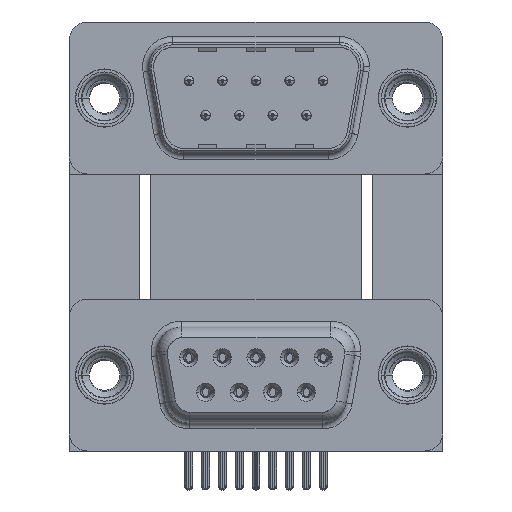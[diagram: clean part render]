
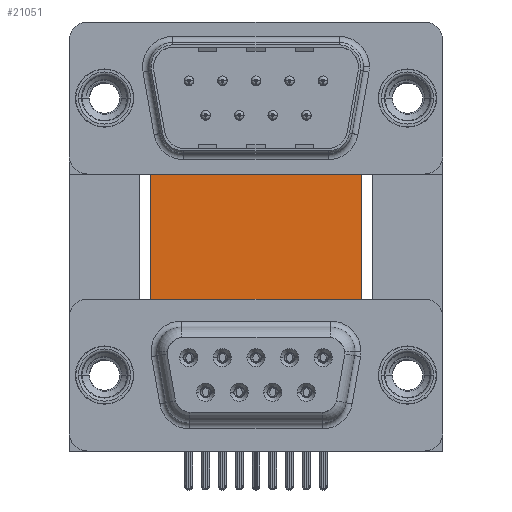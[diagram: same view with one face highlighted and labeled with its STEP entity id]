
A CAD part, top view. The second image highlights one B-rep face of the part: STEP entity #21051.
In plain terms, the highlighted planar face has unit normal (0, 0, 1).
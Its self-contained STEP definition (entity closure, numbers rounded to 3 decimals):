
#100 = CARTESIAN_POINT ( 'NONE',  ( 2.9, -4.635, -12. ) ) ;
#106 = CARTESIAN_POINT ( 'NONE',  ( 3.79, 16.585, -12. ) ) ;
#750 = DIRECTION ( 'NONE',  ( 0., -1., 0. ) ) ;
#1972 = VECTOR ( 'NONE', #31775, 1000. ) ;
#2563 = CARTESIAN_POINT ( 'NONE',  ( 2.9, -3.735, -12. ) ) ;
#2708 = ORIENTED_EDGE ( 'NONE', *, *, #14557, .T. ) ;
#3230 = VERTEX_POINT ( 'NONE', #12802 ) ;
#3780 = CARTESIAN_POINT ( 'NONE',  ( 2.4, -4.635, -12. ) ) ;
#4339 = EDGE_CURVE ( 'NONE', #21287, #3230, #24736, .T. ) ;
#4658 = VERTEX_POINT ( 'NONE', #9778 ) ;
#4846 = ORIENTED_EDGE ( 'NONE', *, *, #35464, .T. ) ;
#4926 = ORIENTED_EDGE ( 'NONE', *, *, #8137, .T. ) ;
#5396 = ORIENTED_EDGE ( 'NONE', *, *, #4339, .T. ) ;
#5978 = LINE ( 'NONE', #2563, #14419 ) ;
#6775 = VECTOR ( 'NONE', #12324, 1000. ) ;
#6816 = LINE ( 'NONE', #31096, #19218 ) ;
#8137 = EDGE_CURVE ( 'NONE', #31065, #26013, #6816, .T. ) ;
#9492 = CARTESIAN_POINT ( 'NONE',  ( 22.59, -4.635, -12. ) ) ;
#9617 = ORIENTED_EDGE ( 'NONE', *, *, #27526, .T. ) ;
#9778 = CARTESIAN_POINT ( 'NONE',  ( 2.9, -4.635, -12. ) ) ;
#10351 = DIRECTION ( 'NONE',  ( 1., 0., 0. ) ) ;
#10736 = CARTESIAN_POINT ( 'NONE',  ( 22.09, -4.635, -12. ) ) ;
#11557 = VECTOR ( 'NONE', #13784, 1000. ) ;
#11712 = VECTOR ( 'NONE', #22302, 1000. ) ;
#11933 = CARTESIAN_POINT ( 'NONE',  ( 2.4, -4.635, -12. ) ) ;
#12324 = DIRECTION ( 'NONE',  ( 1., 0., 0. ) ) ;
#12438 = ORIENTED_EDGE ( 'NONE', *, *, #38053, .T. ) ;
#12591 = LINE ( 'NONE', #24847, #18218 ) ;
#12709 = LINE ( 'NONE', #11933, #30354 ) ;
#12802 = CARTESIAN_POINT ( 'NONE',  ( 21.2, -0.735, -12. ) ) ;
#13046 = CARTESIAN_POINT ( 'NONE',  ( 3.79, 16.585, -12. ) ) ;
#13784 = DIRECTION ( 'NONE',  ( 1., 0., 0. ) ) ;
#14419 = VECTOR ( 'NONE', #18219, 1000. ) ;
#14557 = EDGE_CURVE ( 'NONE', #25342, #37875, #18896, .T. ) ;
#15032 = EDGE_CURVE ( 'NONE', #37875, #33073, #12709, .T. ) ;
#17318 = CARTESIAN_POINT ( 'NONE',  ( 22.59, -4.635, -12. ) ) ;
#18032 = CARTESIAN_POINT ( 'NONE',  ( 3.79, -0.735, -12. ) ) ;
#18116 = EDGE_CURVE ( 'NONE', #33073, #4658, #31199, .T. ) ;
#18166 = CARTESIAN_POINT ( 'NONE',  ( 3.79, 16.585, -12. ) ) ;
#18218 = VECTOR ( 'NONE', #750, 1000. ) ;
#18219 = DIRECTION ( 'NONE',  ( 0., 1., 0. ) ) ;
#18896 = LINE ( 'NONE', #13046, #11712 ) ;
#18967 = FACE_OUTER_BOUND ( 'NONE', #19259, .T. ) ;
#19218 = VECTOR ( 'NONE', #27904, 1000. ) ;
#19259 = EDGE_LOOP ( 'NONE', ( #4926, #12438, #9617, #5396, #25117, #34548, #2708, #35715, #38772, #4846 ) ) ;
#19920 = CARTESIAN_POINT ( 'NONE',  ( 21.2, 16.585, -12. ) ) ;
#21051 = ADVANCED_FACE ( 'NONE', ( #18967 ), #25171, .F. ) ;
#21287 = VERTEX_POINT ( 'NONE', #17318 ) ;
#21584 = DIRECTION ( 'NONE',  ( -1., 0., 0. ) ) ;
#21736 = VERTEX_POINT ( 'NONE', #35579 ) ;
#22302 = DIRECTION ( 'NONE',  ( 0., -1., 0. ) ) ;
#22831 = LINE ( 'NONE', #35298, #11557 ) ;
#24736 = LINE ( 'NONE', #9492, #31613 ) ;
#24847 = CARTESIAN_POINT ( 'NONE',  ( 22.09, -3.735, -12. ) ) ;
#25117 = ORIENTED_EDGE ( 'NONE', *, *, #28380, .F. ) ;
#25171 = PLANE ( 'NONE',  #37101 ) ;
#25342 = VERTEX_POINT ( 'NONE', #18166 ) ;
#25664 = VECTOR ( 'NONE', #10351, 1000. ) ;
#26013 = VERTEX_POINT ( 'NONE', #37363 ) ;
#27526 = EDGE_CURVE ( 'NONE', #21736, #21287, #37870, .T. ) ;
#27616 = DIRECTION ( 'NONE',  ( 0., 0., -1. ) ) ;
#27904 = DIRECTION ( 'NONE',  ( 1., 0., 0. ) ) ;
#28076 = EDGE_CURVE ( 'NONE', #25342, #28505, #22831, .T. ) ;
#28380 = EDGE_CURVE ( 'NONE', #28505, #3230, #34608, .T. ) ;
#28505 = VERTEX_POINT ( 'NONE', #30133 ) ;
#28856 = CARTESIAN_POINT ( 'NONE',  ( 2.9, -3.735, -12. ) ) ;
#30133 = CARTESIAN_POINT ( 'NONE',  ( 21.2, 16.585, -12. ) ) ;
#30354 = VECTOR ( 'NONE', #36663, 1000. ) ;
#31065 = VERTEX_POINT ( 'NONE', #28856 ) ;
#31096 = CARTESIAN_POINT ( 'NONE',  ( 3.79, -3.735, -12. ) ) ;
#31199 = LINE ( 'NONE', #100, #6775 ) ;
#31613 = VECTOR ( 'NONE', #37027, 1000. ) ;
#31775 = DIRECTION ( 'NONE',  ( 0., -1., 0. ) ) ;
#33073 = VERTEX_POINT ( 'NONE', #3780 ) ;
#34548 = ORIENTED_EDGE ( 'NONE', *, *, #28076, .F. ) ;
#34608 = LINE ( 'NONE', #19920, #1972 ) ;
#35298 = CARTESIAN_POINT ( 'NONE',  ( 3.79, 16.585, -12. ) ) ;
#35464 = EDGE_CURVE ( 'NONE', #4658, #31065, #5978, .T. ) ;
#35579 = CARTESIAN_POINT ( 'NONE',  ( 22.09, -4.635, -12. ) ) ;
#35715 = ORIENTED_EDGE ( 'NONE', *, *, #15032, .T. ) ;
#36663 = DIRECTION ( 'NONE',  ( -0.336, -0.942, 0. ) ) ;
#37027 = DIRECTION ( 'NONE',  ( -0.336, 0.942, 0. ) ) ;
#37101 = AXIS2_PLACEMENT_3D ( 'NONE', #106, #27616, #21584 ) ;
#37363 = CARTESIAN_POINT ( 'NONE',  ( 22.09, -3.735, -12. ) ) ;
#37870 = LINE ( 'NONE', #10736, #25664 ) ;
#37875 = VERTEX_POINT ( 'NONE', #18032 ) ;
#38053 = EDGE_CURVE ( 'NONE', #26013, #21736, #12591, .T. ) ;
#38772 = ORIENTED_EDGE ( 'NONE', *, *, #18116, .T. ) ;
